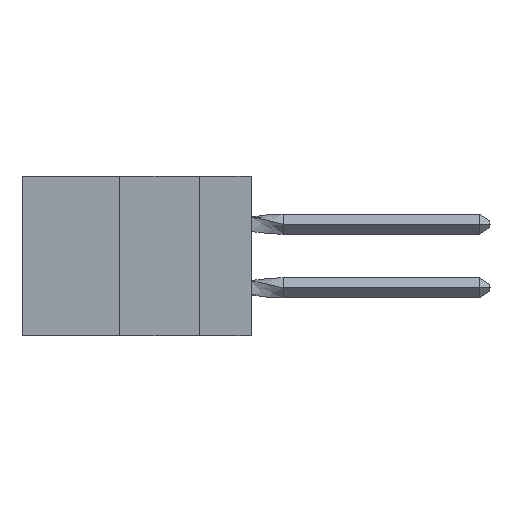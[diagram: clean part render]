
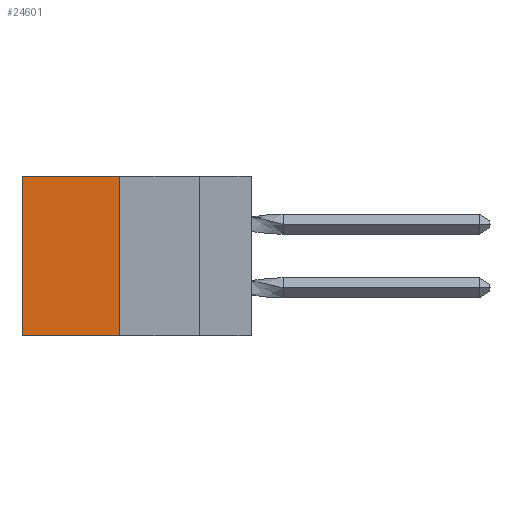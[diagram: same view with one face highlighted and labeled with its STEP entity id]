
A CAD part, left-side view. The second image highlights one B-rep face of the part: STEP entity #24601.
In plain terms, the highlighted planar face has unit normal (-1, 0, 0).
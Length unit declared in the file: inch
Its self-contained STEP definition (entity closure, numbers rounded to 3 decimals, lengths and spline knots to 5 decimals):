
#42 = EDGE_LOOP ( 'NONE', ( #20184, #13476, #10366, #2629 ) ) ;
#164 = CARTESIAN_POINT ( 'NONE',  ( 0.305, 0.72, -0.5 ) ) ;
#422 = DIRECTION ( 'NONE',  ( 0., 1., 0. ) ) ;
#1354 = DIRECTION ( 'NONE',  ( 0., 0., -1. ) ) ;
#1442 = CARTESIAN_POINT ( 'NONE',  ( 0.305, 0.413, -0.5 ) ) ;
#1812 = LINE ( 'NONE', #1442, #17587 ) ;
#1939 = LINE ( 'NONE', #11277, #11226 ) ;
#2482 = DIRECTION ( 'NONE',  ( 1., 0., 0. ) ) ;
#2629 = ORIENTED_EDGE ( 'NONE', *, *, #10751, .T. ) ;
#6824 = LINE ( 'NONE', #11478, #7179 ) ;
#7070 = CARTESIAN_POINT ( 'NONE',  ( 0.305, 0.413, -0.5 ) ) ;
#7178 = DIRECTION ( 'NONE',  ( 0., 0., -1. ) ) ;
#7179 = VECTOR ( 'NONE', #7235, 39.37008 ) ;
#7235 = DIRECTION ( 'NONE',  ( 0., 1., 0. ) ) ;
#8628 = EDGE_CURVE ( 'NONE', #12476, #23953, #1812, .T. ) ;
#10366 = ORIENTED_EDGE ( 'NONE', *, *, #8628, .F. ) ;
#10751 = EDGE_CURVE ( 'NONE', #12476, #18140, #6824, .T. ) ;
#10869 = DIRECTION ( 'NONE',  ( 0., 0., -1. ) ) ;
#11081 = CARTESIAN_POINT ( 'NONE',  ( 0.305, 0.413, -0.5 ) ) ;
#11226 = VECTOR ( 'NONE', #422, 39.37008 ) ;
#11277 = CARTESIAN_POINT ( 'NONE',  ( 0.305, 0.413, -0.5 ) ) ;
#11478 = CARTESIAN_POINT ( 'NONE',  ( 0.305, 0.413, 0. ) ) ;
#12476 = VERTEX_POINT ( 'NONE', #26101 ) ;
#12647 = VERTEX_POINT ( 'NONE', #164 ) ;
#12691 = FACE_OUTER_BOUND ( 'NONE', #42, .T. ) ;
#13476 = ORIENTED_EDGE ( 'NONE', *, *, #27197, .F. ) ;
#15245 = LINE ( 'NONE', #28287, #23151 ) ;
#17587 = VECTOR ( 'NONE', #1354, 39.37008 ) ;
#18140 = VERTEX_POINT ( 'NONE', #21480 ) ;
#18784 = AXIS2_PLACEMENT_3D ( 'NONE', #7070, #2482, #7178 ) ;
#20184 = ORIENTED_EDGE ( 'NONE', *, *, #20497, .T. ) ;
#20497 = EDGE_CURVE ( 'NONE', #18140, #12647, #15245, .T. ) ;
#21480 = CARTESIAN_POINT ( 'NONE',  ( 0.305, 0.72, 0. ) ) ;
#23151 = VECTOR ( 'NONE', #10869, 39.37008 ) ;
#23953 = VERTEX_POINT ( 'NONE', #11081 ) ;
#24601 = ADVANCED_FACE ( 'NONE', ( #12691 ), #24611, .F. ) ;
#24611 = PLANE ( 'NONE',  #18784 ) ;
#26101 = CARTESIAN_POINT ( 'NONE',  ( 0.305, 0.413, 0. ) ) ;
#27197 = EDGE_CURVE ( 'NONE', #23953, #12647, #1939, .T. ) ;
#28287 = CARTESIAN_POINT ( 'NONE',  ( 0.305, 0.72, -0.5 ) ) ;
